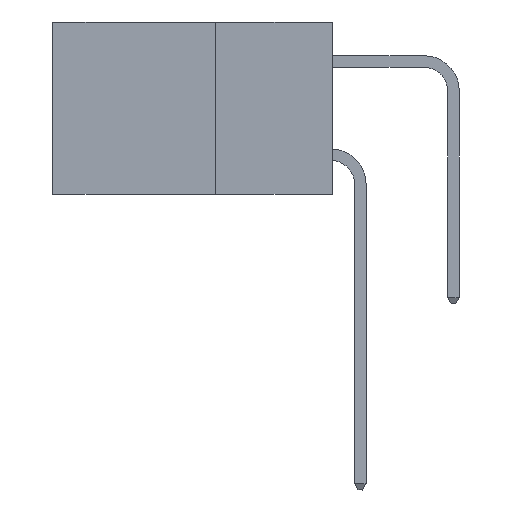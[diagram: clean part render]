
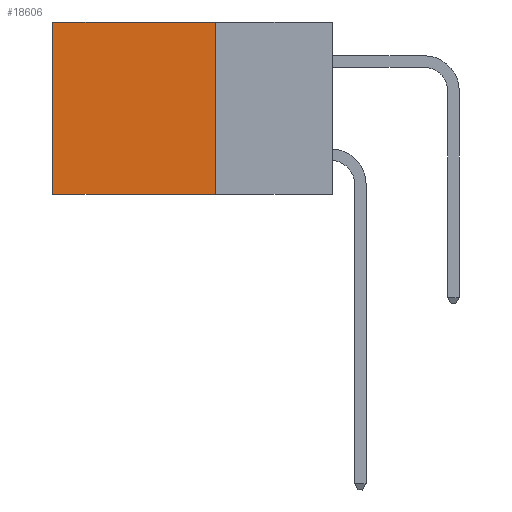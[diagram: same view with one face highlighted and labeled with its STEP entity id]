
A CAD part, left-side view. The second image highlights one B-rep face of the part: STEP entity #18606.
In plain terms, the highlighted planar face has unit normal (-1, 0, 0).
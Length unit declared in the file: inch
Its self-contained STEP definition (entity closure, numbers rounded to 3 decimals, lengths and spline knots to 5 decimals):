
#437 = LINE ( 'NONE', #20803, #17875 ) ;
#1798 = CARTESIAN_POINT ( 'NONE',  ( 0.2615, 0.25, 0. ) ) ;
#1910 = PLANE ( 'NONE',  #10034 ) ;
#2340 = ORIENTED_EDGE ( 'NONE', *, *, #24020, .T. ) ;
#3671 = VERTEX_POINT ( 'NONE', #18063 ) ;
#3997 = CARTESIAN_POINT ( 'NONE',  ( 0.2615, 0.25, -0.37 ) ) ;
#4567 = EDGE_CURVE ( 'NONE', #3671, #11511, #23994, .T. ) ;
#4948 = CARTESIAN_POINT ( 'NONE',  ( 0.2615, 0.25, 0. ) ) ;
#5603 = LINE ( 'NONE', #7325, #22181 ) ;
#6076 = EDGE_LOOP ( 'NONE', ( #15557, #12657, #16080, #2340 ) ) ;
#6972 = LINE ( 'NONE', #1798, #14807 ) ;
#6974 = VERTEX_POINT ( 'NONE', #4948 ) ;
#7325 = CARTESIAN_POINT ( 'NONE',  ( 0.2615, 0.25, -0.37 ) ) ;
#7444 = FACE_OUTER_BOUND ( 'NONE', #6076, .T. ) ;
#7933 = DIRECTION ( 'NONE',  ( 0., 1., 0. ) ) ;
#9163 = CARTESIAN_POINT ( 'NONE',  ( 0.2615, 0.6, -0.37 ) ) ;
#9430 = CARTESIAN_POINT ( 'NONE',  ( 0.2615, 0.6, -0.37 ) ) ;
#10034 = AXIS2_PLACEMENT_3D ( 'NONE', #3997, #15139, #14902 ) ;
#11511 = VERTEX_POINT ( 'NONE', #9430 ) ;
#12657 = ORIENTED_EDGE ( 'NONE', *, *, #21324, .F. ) ;
#13079 = CARTESIAN_POINT ( 'NONE',  ( 0.2615, 0.25, -0.37 ) ) ;
#13654 = VERTEX_POINT ( 'NONE', #13079 ) ;
#14807 = VECTOR ( 'NONE', #23887, 39.37008 ) ;
#14902 = DIRECTION ( 'NONE',  ( 0., 0., -1. ) ) ;
#15139 = DIRECTION ( 'NONE',  ( 1., 0., 0. ) ) ;
#15557 = ORIENTED_EDGE ( 'NONE', *, *, #4567, .T. ) ;
#16080 = ORIENTED_EDGE ( 'NONE', *, *, #21074, .F. ) ;
#17875 = VECTOR ( 'NONE', #7933, 39.37008 ) ;
#18063 = CARTESIAN_POINT ( 'NONE',  ( 0.2615, 0.6, 0. ) ) ;
#18334 = DIRECTION ( 'NONE',  ( 0., 0., -1. ) ) ;
#18459 = DIRECTION ( 'NONE',  ( 0., 0., -1. ) ) ;
#18606 = ADVANCED_FACE ( 'NONE', ( #7444 ), #1910, .F. ) ;
#19227 = VECTOR ( 'NONE', #18459, 39.37008 ) ;
#20803 = CARTESIAN_POINT ( 'NONE',  ( 0.2615, 0.25, -0.37 ) ) ;
#21074 = EDGE_CURVE ( 'NONE', #6974, #13654, #5603, .T. ) ;
#21324 = EDGE_CURVE ( 'NONE', #13654, #11511, #437, .T. ) ;
#22181 = VECTOR ( 'NONE', #18334, 39.37008 ) ;
#23887 = DIRECTION ( 'NONE',  ( 0., 1., 0. ) ) ;
#23994 = LINE ( 'NONE', #9163, #19227 ) ;
#24020 = EDGE_CURVE ( 'NONE', #6974, #3671, #6972, .T. ) ;
